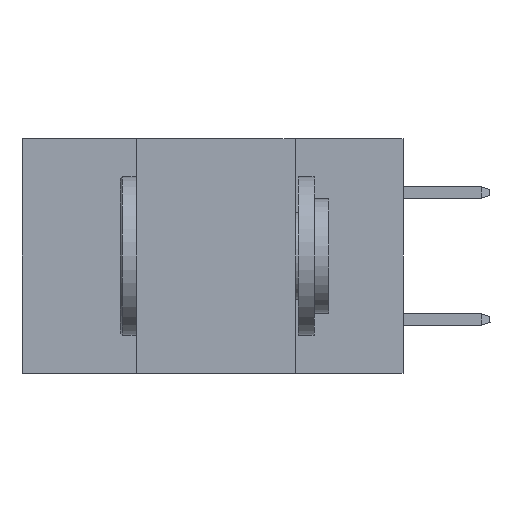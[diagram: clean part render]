
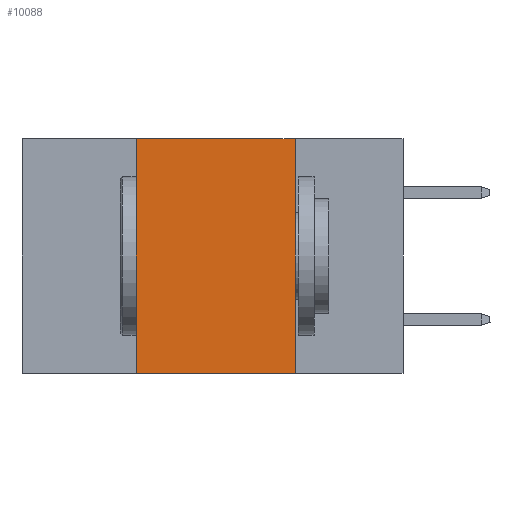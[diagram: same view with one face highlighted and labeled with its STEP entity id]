
A CAD part, left-side view. The second image highlights one B-rep face of the part: STEP entity #10088.
In plain terms, the highlighted planar face has unit normal (-1, 0, 0).
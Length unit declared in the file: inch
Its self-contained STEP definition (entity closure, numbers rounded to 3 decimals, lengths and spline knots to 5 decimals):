
#245 = CARTESIAN_POINT ( 'NONE',  ( 0., 0.42, -0.37 ) ) ;
#314 = PLANE ( 'NONE',  #20103 ) ;
#814 = DIRECTION ( 'NONE',  ( 0., 0., -1. ) ) ;
#920 = VECTOR ( 'NONE', #2519, 39.37008 ) ;
#1049 = EDGE_LOOP ( 'NONE', ( #19412, #20615, #9506, #11335 ) ) ;
#1945 = EDGE_CURVE ( 'NONE', #2702, #6381, #18962, .T. ) ;
#2519 = DIRECTION ( 'NONE',  ( 0., -1., 0. ) ) ;
#2702 = VERTEX_POINT ( 'NONE', #12841 ) ;
#3982 = CARTESIAN_POINT ( 'NONE',  ( 0., 0.42, 0. ) ) ;
#6381 = VERTEX_POINT ( 'NONE', #20314 ) ;
#6877 = CARTESIAN_POINT ( 'NONE',  ( 0., 0.6, 0. ) ) ;
#7826 = LINE ( 'NONE', #15315, #920 ) ;
#7973 = EDGE_CURVE ( 'NONE', #15561, #22347, #19245, .T. ) ;
#9506 = ORIENTED_EDGE ( 'NONE', *, *, #7973, .F. ) ;
#9784 = DIRECTION ( 'NONE',  ( 0., 0., -1. ) ) ;
#10088 = ADVANCED_FACE ( 'NONE', ( #16564 ), #314, .F. ) ;
#11260 = CARTESIAN_POINT ( 'NONE',  ( 0., 0.17, 0. ) ) ;
#11335 = ORIENTED_EDGE ( 'NONE', *, *, #16977, .T. ) ;
#11760 = CARTESIAN_POINT ( 'NONE',  ( 0., 0.42, 0. ) ) ;
#12841 = CARTESIAN_POINT ( 'NONE',  ( 0., 0.17, 0. ) ) ;
#15315 = CARTESIAN_POINT ( 'NONE',  ( 0., 0.6, -0.37 ) ) ;
#15561 = VERTEX_POINT ( 'NONE', #245 ) ;
#15798 = EDGE_CURVE ( 'NONE', #22347, #2702, #15909, .T. ) ;
#15909 = LINE ( 'NONE', #6877, #18451 ) ;
#16345 = DIRECTION ( 'NONE',  ( 1., 0., 0. ) ) ;
#16564 = FACE_OUTER_BOUND ( 'NONE', #1049, .T. ) ;
#16977 = EDGE_CURVE ( 'NONE', #15561, #6381, #7826, .T. ) ;
#17328 = DIRECTION ( 'NONE',  ( 0., -1., 0. ) ) ;
#18121 = CARTESIAN_POINT ( 'NONE',  ( 0., 0.6, 0. ) ) ;
#18139 = VECTOR ( 'NONE', #20673, 39.37008 ) ;
#18451 = VECTOR ( 'NONE', #17328, 39.37008 ) ;
#18962 = LINE ( 'NONE', #11260, #22900 ) ;
#19245 = LINE ( 'NONE', #11760, #18139 ) ;
#19412 = ORIENTED_EDGE ( 'NONE', *, *, #1945, .F. ) ;
#20103 = AXIS2_PLACEMENT_3D ( 'NONE', #18121, #16345, #9784 ) ;
#20314 = CARTESIAN_POINT ( 'NONE',  ( 0., 0.17, -0.37 ) ) ;
#20615 = ORIENTED_EDGE ( 'NONE', *, *, #15798, .F. ) ;
#20673 = DIRECTION ( 'NONE',  ( 0., 0., 1. ) ) ;
#22347 = VERTEX_POINT ( 'NONE', #3982 ) ;
#22900 = VECTOR ( 'NONE', #814, 39.37008 ) ;
